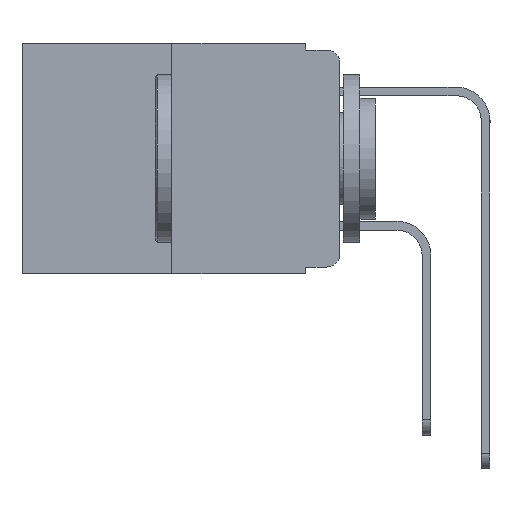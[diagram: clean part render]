
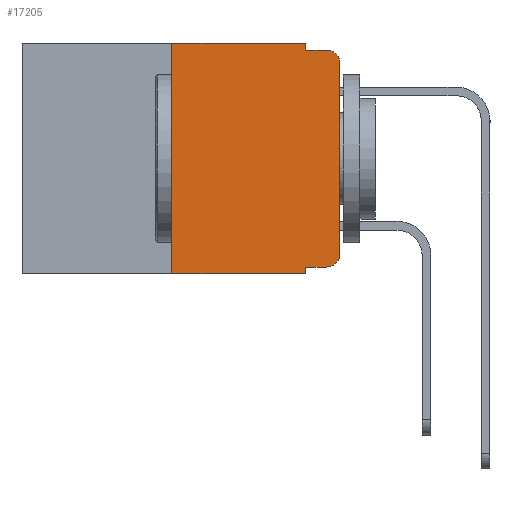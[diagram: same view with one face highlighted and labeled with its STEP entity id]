
A CAD part, left-side view. The second image highlights one B-rep face of the part: STEP entity #17205.
In plain terms, the highlighted planar face has unit normal (-1, 0, 0).
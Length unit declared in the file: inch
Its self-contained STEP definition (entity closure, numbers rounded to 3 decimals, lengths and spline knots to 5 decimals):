
#74 = CARTESIAN_POINT ( 'NONE',  ( 0., 0.25, 0. ) ) ;
#365 = CARTESIAN_POINT ( 'NONE',  ( 0., 0.051, -0.333 ) ) ;
#773 = VECTOR ( 'NONE', #1109, 39.37008 ) ;
#1109 = DIRECTION ( 'NONE',  ( 0., -1., 0. ) ) ;
#1199 = EDGE_CURVE ( 'NONE', #10713, #15744, #7199, .T. ) ;
#1230 = CARTESIAN_POINT ( 'NONE',  ( 0., 0.473, -0.343 ) ) ;
#1880 = CARTESIAN_POINT ( 'NONE',  ( 0., 0.473, 0. ) ) ;
#2314 = DIRECTION ( 'NONE',  ( 1., 0., 0. ) ) ;
#2317 = EDGE_CURVE ( 'NONE', #12283, #10713, #9905, .T. ) ;
#2774 = VECTOR ( 'NONE', #11191, 39.37008 ) ;
#3538 = CARTESIAN_POINT ( 'NONE',  ( 0., 0., -0.313 ) ) ;
#3713 = CARTESIAN_POINT ( 'NONE',  ( 0., 0., -0.03 ) ) ;
#4108 = DIRECTION ( 'NONE',  ( 0., 0., -1. ) ) ;
#4578 = DIRECTION ( 'NONE',  ( 0., -1., 0. ) ) ;
#4913 = VECTOR ( 'NONE', #19032, 39.37008 ) ;
#4927 = ORIENTED_EDGE ( 'NONE', *, *, #5800, .F. ) ;
#5115 = CARTESIAN_POINT ( 'NONE',  ( 0., 0.02, -0.333 ) ) ;
#5551 = VERTEX_POINT ( 'NONE', #74 ) ;
#5555 = CARTESIAN_POINT ( 'NONE',  ( 0., 0.051, 0. ) ) ;
#5646 = EDGE_CURVE ( 'NONE', #12283, #16706, #10787, .T. ) ;
#5704 = VECTOR ( 'NONE', #4578, 39.37008 ) ;
#5800 = EDGE_CURVE ( 'NONE', #5551, #15691, #19653, .T. ) ;
#5816 = VERTEX_POINT ( 'NONE', #17675 ) ;
#5917 = ORIENTED_EDGE ( 'NONE', *, *, #12993, .F. ) ;
#6163 = CARTESIAN_POINT ( 'NONE',  ( 0., 0.051, -0.333 ) ) ;
#6675 = DIRECTION ( 'NONE',  ( 0., -1., 0. ) ) ;
#6678 = EDGE_CURVE ( 'NONE', #13277, #5551, #20063, .T. ) ;
#6965 = VECTOR ( 'NONE', #6675, 39.37008 ) ;
#7143 = CARTESIAN_POINT ( 'NONE',  ( 0., 0.02, -0.03 ) ) ;
#7199 = CIRCLE ( 'NONE', #18175, 0.02 ) ;
#7254 = CARTESIAN_POINT ( 'NONE',  ( 0., 0.051, -0.343 ) ) ;
#7285 = VERTEX_POINT ( 'NONE', #18566 ) ;
#7736 = EDGE_CURVE ( 'NONE', #15691, #7285, #13127, .T. ) ;
#7809 = VECTOR ( 'NONE', #8336, 39.37008 ) ;
#7901 = EDGE_LOOP ( 'NONE', ( #20370, #9134, #5917, #19706, #4927, #10612, #18785, #20168, #16904, #18804 ) ) ;
#8238 = CARTESIAN_POINT ( 'NONE',  ( 0., 0., 0. ) ) ;
#8336 = DIRECTION ( 'NONE',  ( 0., -1., 0. ) ) ;
#8779 = DIRECTION ( 'NONE',  ( 0., 0., -1. ) ) ;
#9134 = ORIENTED_EDGE ( 'NONE', *, *, #14029, .T. ) ;
#9176 = CIRCLE ( 'NONE', #9740, 0.02 ) ;
#9364 = CARTESIAN_POINT ( 'NONE',  ( 0., 0.02, -0.313 ) ) ;
#9419 = LINE ( 'NONE', #1230, #5704 ) ;
#9673 = DIRECTION ( 'NONE',  ( 0., 0., -1. ) ) ;
#9734 = DIRECTION ( 'NONE',  ( -1., 0., 0. ) ) ;
#9740 = AXIS2_PLACEMENT_3D ( 'NONE', #7143, #18009, #8779 ) ;
#9905 = LINE ( 'NONE', #365, #773 ) ;
#10121 = VERTEX_POINT ( 'NONE', #3713 ) ;
#10612 = ORIENTED_EDGE ( 'NONE', *, *, #6678, .F. ) ;
#10713 = VERTEX_POINT ( 'NONE', #5115 ) ;
#10787 = LINE ( 'NONE', #5555, #2774 ) ;
#11154 = LINE ( 'NONE', #16033, #6965 ) ;
#11191 = DIRECTION ( 'NONE',  ( 0., 0., -1. ) ) ;
#11316 = LINE ( 'NONE', #8238, #4913 ) ;
#12283 = VERTEX_POINT ( 'NONE', #6163 ) ;
#12389 = DIRECTION ( 'NONE',  ( 0., 0., 1. ) ) ;
#12993 = EDGE_CURVE ( 'NONE', #7285, #5816, #11154, .T. ) ;
#13127 = LINE ( 'NONE', #13510, #17208 ) ;
#13277 = VERTEX_POINT ( 'NONE', #18003 ) ;
#13376 = CARTESIAN_POINT ( 'NONE',  ( 0., 0.473, 0. ) ) ;
#13439 = DIRECTION ( 'NONE',  ( 0., 0., -1. ) ) ;
#13510 = CARTESIAN_POINT ( 'NONE',  ( 0., 0.051, 0. ) ) ;
#14029 = EDGE_CURVE ( 'NONE', #10121, #5816, #9176, .T. ) ;
#14214 = CARTESIAN_POINT ( 'NONE',  ( 0., 0.25, 0. ) ) ;
#14313 = EDGE_CURVE ( 'NONE', #13277, #16706, #9419, .T. ) ;
#14374 = CARTESIAN_POINT ( 'NONE',  ( 0., 0.051, 0. ) ) ;
#15078 = EDGE_CURVE ( 'NONE', #15744, #10121, #11316, .T. ) ;
#15691 = VERTEX_POINT ( 'NONE', #14374 ) ;
#15744 = VERTEX_POINT ( 'NONE', #3538 ) ;
#16033 = CARTESIAN_POINT ( 'NONE',  ( 0., 0.051, -0.01 ) ) ;
#16077 = VECTOR ( 'NONE', #12389, 39.37008 ) ;
#16706 = VERTEX_POINT ( 'NONE', #7254 ) ;
#16904 = ORIENTED_EDGE ( 'NONE', *, *, #2317, .T. ) ;
#17205 = ADVANCED_FACE ( 'NONE', ( #18200 ), #17992, .F. ) ;
#17208 = VECTOR ( 'NONE', #4108, 39.37008 ) ;
#17273 = AXIS2_PLACEMENT_3D ( 'NONE', #13376, #2314, #13439 ) ;
#17675 = CARTESIAN_POINT ( 'NONE',  ( 0., 0.02, -0.01 ) ) ;
#17992 = PLANE ( 'NONE',  #17273 ) ;
#18003 = CARTESIAN_POINT ( 'NONE',  ( 0., 0.25, -0.343 ) ) ;
#18009 = DIRECTION ( 'NONE',  ( -1., 0., 0. ) ) ;
#18175 = AXIS2_PLACEMENT_3D ( 'NONE', #9364, #9734, #9673 ) ;
#18200 = FACE_OUTER_BOUND ( 'NONE', #7901, .T. ) ;
#18566 = CARTESIAN_POINT ( 'NONE',  ( 0., 0.051, -0.01 ) ) ;
#18785 = ORIENTED_EDGE ( 'NONE', *, *, #14313, .T. ) ;
#18804 = ORIENTED_EDGE ( 'NONE', *, *, #1199, .T. ) ;
#19032 = DIRECTION ( 'NONE',  ( 0., 0., 1. ) ) ;
#19653 = LINE ( 'NONE', #1880, #7809 ) ;
#19706 = ORIENTED_EDGE ( 'NONE', *, *, #7736, .F. ) ;
#20063 = LINE ( 'NONE', #14214, #16077 ) ;
#20168 = ORIENTED_EDGE ( 'NONE', *, *, #5646, .F. ) ;
#20370 = ORIENTED_EDGE ( 'NONE', *, *, #15078, .T. ) ;
